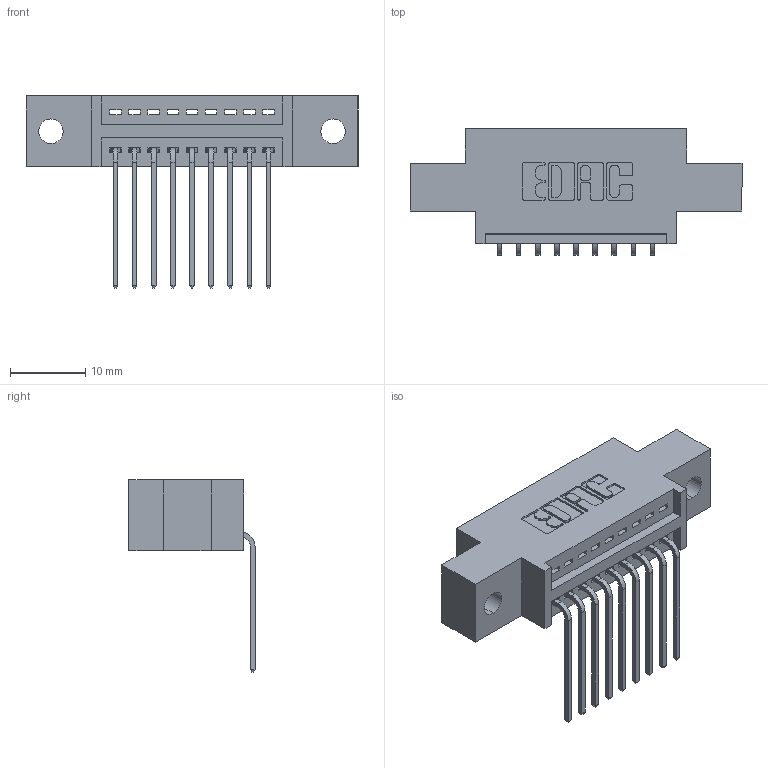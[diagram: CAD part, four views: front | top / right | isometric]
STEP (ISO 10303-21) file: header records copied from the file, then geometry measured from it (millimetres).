
FILE_DESCRIPTION (( 'STEP AP203' ), '1' );
FILE_NAME ('395-009-559-602.STEP', '2019-10-15T20:56:39', ( '' ), ( '' ), 'SwSTEP 2.0', 'SolidWorks 2016', '' );
FILE_SCHEMA (( 'CONFIG_CONTROL_DESIGN' ));
Length unit declared in the file: inch
Products named in the file (3): 395-009-559-602; 345-292-001_558 559 Tail - 1; 345 Part_0.170 Offset - 0.128 Dia
Assembly tree (10 placements, depth 2):
  395-009-559-602
    345 Part_0.170 Offset - 0.128 Dia
    345-292-001_558 559 Tail - 1  x9
Bounding box: 44.07 x 16.75 x 25.53 mm (x, y, z)
Volume: 3795.3 mm3; surface area: 4626.4 mm2
Topology: 10 solids, 10 shells, 670 faces, 1991 edges, 1314 vertices
Faces by surface type: plane 462, cylinder 208
Entity records: 11435 total; most frequent: CARTESIAN_POINT 1991, ORIENTED_EDGE 1934, DIRECTION 1785, EDGE_CURVE 967, LINE 799, VECTOR 799, VERTEX_POINT 642, AXIS2_PLACEMENT_3D 493
